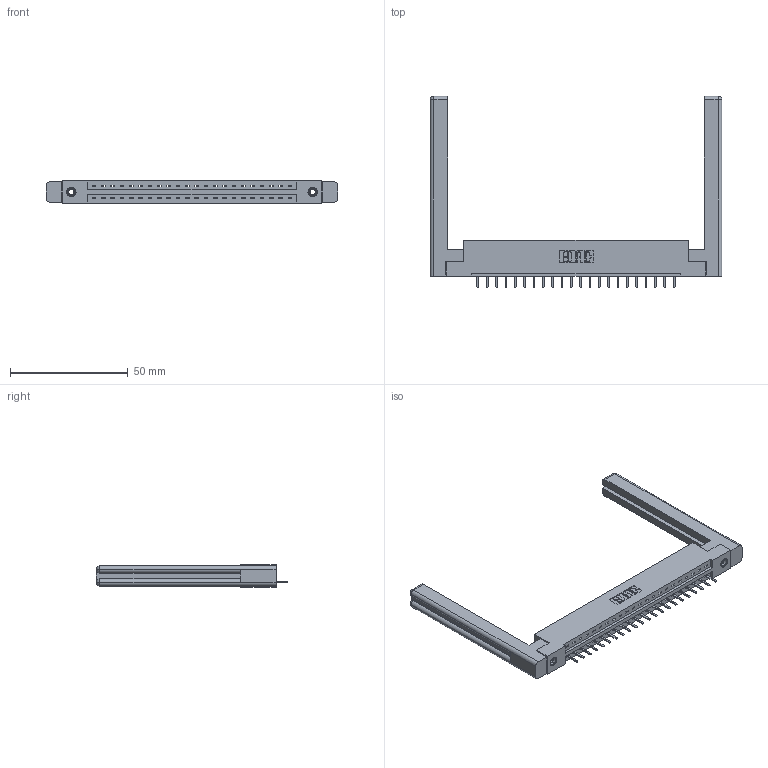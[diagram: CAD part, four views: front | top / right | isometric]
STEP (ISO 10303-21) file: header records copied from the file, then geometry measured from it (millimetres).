
FILE_DESCRIPTION (( 'STEP AP203' ), '1' );
FILE_NAME ('387-022-520-158.STEP', '2019-10-03T00:43:24', ( '' ), ( '' ), 'SwSTEP 2.0', 'SolidWorks 2016', '' );
FILE_SCHEMA (( 'CONFIG_CONTROL_DESIGN' ));
Length unit declared in the file: inch
Products named in the file (5): 345-292-001_345-293-120; 337 Part_Flush Mounting Lugs - 0.156 Dia-TI; 307-220-058; 345-250-001_345-250-001-102; 387-022-520-158
Assembly tree (27 placements, depth 2):
  387-022-520-158
    337 Part_Flush Mounting Lugs - 0.156 Dia-TI
    345-292-001_345-293-120  x22
    345-250-001_345-250-001-102  x2
    307-220-058  x2
Bounding box: 123.8 x 81.11 x 9.4 mm (x, y, z)
Volume: 19715.5 mm3; surface area: 17846.2 mm2
Topology: 27 solids, 27 shells, 1708 faces, 4977 edges, 3246 vertices
Faces by surface type: plane 1210, cylinder 474, cone 12, torus 12
Entity records: 21688 total; most frequent: CARTESIAN_POINT 3787, ORIENTED_EDGE 3672, DIRECTION 3236, EDGE_CURVE 1836, VECTOR 1656, LINE 1656, VERTEX_POINT 1214, AXIS2_PLACEMENT_3D 790
